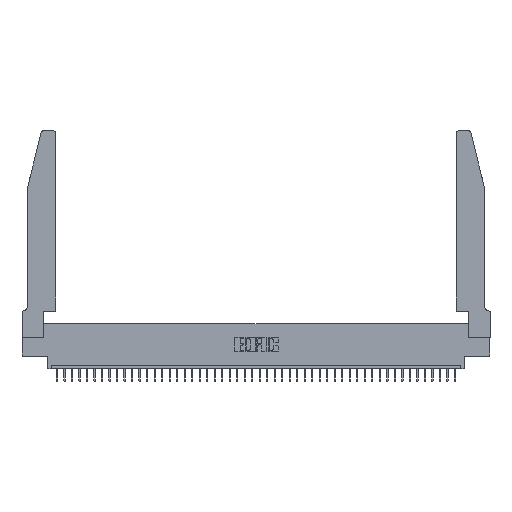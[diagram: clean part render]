
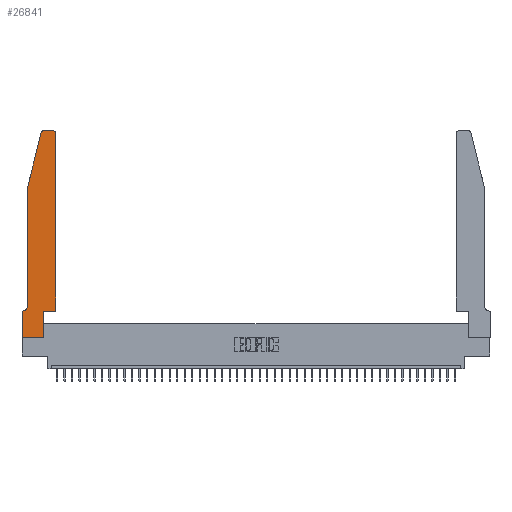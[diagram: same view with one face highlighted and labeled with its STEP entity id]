
A CAD part, top view. The second image highlights one B-rep face of the part: STEP entity #26841.
In plain terms, the highlighted planar face has unit normal (0, 0, 1).
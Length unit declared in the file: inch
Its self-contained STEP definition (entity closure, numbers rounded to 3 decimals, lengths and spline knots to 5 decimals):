
#531 = DIRECTION ( 'NONE',  ( 1., 0., 0. ) ) ;
#1023 = ORIENTED_EDGE ( 'NONE', *, *, #35085, .T. ) ;
#1380 = VERTEX_POINT ( 'NONE', #29385 ) ;
#1399 = VECTOR ( 'NONE', #27630, 39.37008 ) ;
#1460 = CARTESIAN_POINT ( 'NONE',  ( 0.0055, 0.42, 0.37 ) ) ;
#1509 = CARTESIAN_POINT ( 'NONE',  ( 0.284, 2.72, 0.37 ) ) ;
#1550 = CARTESIAN_POINT ( 'NONE',  ( 0.0755, 0.35, 0.37 ) ) ;
#1825 = VECTOR ( 'NONE', #17732, 39.37008 ) ;
#2286 = VERTEX_POINT ( 'NONE', #15661 ) ;
#3077 = CARTESIAN_POINT ( 'NONE',  ( 0.2865, 0.35, 0.37 ) ) ;
#3195 = ORIENTED_EDGE ( 'NONE', *, *, #18714, .T. ) ;
#3375 = ORIENTED_EDGE ( 'NONE', *, *, #33990, .T. ) ;
#3528 = PLANE ( 'NONE',  #32171 ) ;
#4137 = ORIENTED_EDGE ( 'NONE', *, *, #41520, .T. ) ;
#4184 = ORIENTED_EDGE ( 'NONE', *, *, #13365, .T. ) ;
#4264 = VERTEX_POINT ( 'NONE', #23359 ) ;
#4670 = CARTESIAN_POINT ( 'NONE',  ( 0.284, 2.75, 0.37 ) ) ;
#5471 = ORIENTED_EDGE ( 'NONE', *, *, #19715, .T. ) ;
#6332 = VECTOR ( 'NONE', #34596, 39.37008 ) ;
#7125 = EDGE_CURVE ( 'NONE', #2286, #23668, #32924, .T. ) ;
#8430 = DIRECTION ( 'NONE',  ( -1., 0., 0. ) ) ;
#8462 = DIRECTION ( 'NONE',  ( 1., 0., 0. ) ) ;
#10870 = VERTEX_POINT ( 'NONE', #19132 ) ;
#11763 = DIRECTION ( 'NONE',  ( 0., 0., 1. ) ) ;
#12128 = VECTOR ( 'NONE', #14571, 39.37008 ) ;
#12624 = VERTEX_POINT ( 'NONE', #4670 ) ;
#13365 = EDGE_CURVE ( 'NONE', #4264, #10870, #25734, .T. ) ;
#13976 = CARTESIAN_POINT ( 'NONE',  ( 0.2865, 0., 0.37 ) ) ;
#14091 = DIRECTION ( 'NONE',  ( 1., 0., 0. ) ) ;
#14571 = DIRECTION ( 'NONE',  ( 0., 1., 0. ) ) ;
#14810 = VERTEX_POINT ( 'NONE', #31232 ) ;
#14956 = VECTOR ( 'NONE', #15767, 39.37008 ) ;
#15661 = CARTESIAN_POINT ( 'NONE',  ( 0., 0.35, 0.37 ) ) ;
#15767 = DIRECTION ( 'NONE',  ( 0., -1., 0. ) ) ;
#16477 = EDGE_CURVE ( 'NONE', #14810, #12624, #29473, .T. ) ;
#16631 = FACE_OUTER_BOUND ( 'NONE', #20950, .T. ) ;
#17285 = VERTEX_POINT ( 'NONE', #38273 ) ;
#17711 = CARTESIAN_POINT ( 'NONE',  ( 0.4505, 0.35, 0.37 ) ) ;
#17732 = DIRECTION ( 'NONE',  ( -1., 0., 0. ) ) ;
#18138 = CARTESIAN_POINT ( 'NONE',  ( 0.0755, 2., 0.37 ) ) ;
#18714 = EDGE_CURVE ( 'NONE', #17285, #14810, #20323, .T. ) ;
#19132 = CARTESIAN_POINT ( 'NONE',  ( 0.0055, 0.35, 0.37 ) ) ;
#19475 = LINE ( 'NONE', #18138, #24700 ) ;
#19620 = EDGE_CURVE ( 'NONE', #10870, #2286, #42398, .T. ) ;
#19715 = EDGE_CURVE ( 'NONE', #24317, #27236, #36018, .T. ) ;
#20323 = CIRCLE ( 'NONE', #25554, 0.03 ) ;
#20950 = EDGE_LOOP ( 'NONE', ( #22391, #40862, #4137, #21047, #4184, #28801, #35682, #3375, #5471, #30517, #1023, #3195 ) ) ;
#21047 = ORIENTED_EDGE ( 'NONE', *, *, #34521, .T. ) ;
#21108 = CARTESIAN_POINT ( 'NONE',  ( 0.2605, 2.75, 0.37 ) ) ;
#22391 = ORIENTED_EDGE ( 'NONE', *, *, #16477, .T. ) ;
#23034 = CARTESIAN_POINT ( 'NONE',  ( 0.2865, 0.35, 0.37 ) ) ;
#23359 = CARTESIAN_POINT ( 'NONE',  ( 0.0755, 0.42, 0.37 ) ) ;
#23398 = VECTOR ( 'NONE', #14091, 39.37008 ) ;
#23668 = VERTEX_POINT ( 'NONE', #39765 ) ;
#23882 = VECTOR ( 'NONE', #8430, 39.37008 ) ;
#24177 = CARTESIAN_POINT ( 'NONE',  ( 0., 0.35, 0.37 ) ) ;
#24317 = VERTEX_POINT ( 'NONE', #13976 ) ;
#24516 = CARTESIAN_POINT ( 'NONE',  ( 0.4505, 0.35, 0.37 ) ) ;
#24700 = VECTOR ( 'NONE', #31941, 39.37008 ) ;
#25064 = DIRECTION ( 'NONE',  ( -1., 0., 0. ) ) ;
#25554 = AXIS2_PLACEMENT_3D ( 'NONE', #38648, #11763, #8462 ) ;
#25734 = CIRCLE ( 'NONE', #28755, 0.07 ) ;
#25797 = EDGE_CURVE ( 'NONE', #12624, #27061, #40508, .T. ) ;
#26274 = CARTESIAN_POINT ( 'NONE',  ( 0., 0., 0.37 ) ) ;
#26586 = LINE ( 'NONE', #30768, #23398 ) ;
#26841 = ADVANCED_FACE ( 'NONE', ( #16631 ), #3528, .T. ) ;
#27061 = VERTEX_POINT ( 'NONE', #39706 ) ;
#27140 = AXIS2_PLACEMENT_3D ( 'NONE', #1509, #38876, #28854 ) ;
#27236 = VERTEX_POINT ( 'NONE', #3077 ) ;
#27322 = DIRECTION ( 'NONE',  ( 0., 0., 1. ) ) ;
#27356 = CARTESIAN_POINT ( 'NONE',  ( 0.4505, 0.35, 0.37 ) ) ;
#27630 = DIRECTION ( 'NONE',  ( 1., 0., 0. ) ) ;
#28755 = AXIS2_PLACEMENT_3D ( 'NONE', #1460, #37054, #25064 ) ;
#28801 = ORIENTED_EDGE ( 'NONE', *, *, #19620, .T. ) ;
#28854 = DIRECTION ( 'NONE',  ( 1., 0., 0. ) ) ;
#29385 = CARTESIAN_POINT ( 'NONE',  ( 0.0755, 2., 0.37 ) ) ;
#29473 = LINE ( 'NONE', #21108, #1825 ) ;
#30517 = ORIENTED_EDGE ( 'NONE', *, *, #40677, .T. ) ;
#30691 = VECTOR ( 'NONE', #36013, 39.37008 ) ;
#30768 = CARTESIAN_POINT ( 'NONE',  ( 0., 0., 0.37 ) ) ;
#31232 = CARTESIAN_POINT ( 'NONE',  ( 0.4205, 2.75, 0.37 ) ) ;
#31941 = DIRECTION ( 'NONE',  ( -0.239, -0.971, 0. ) ) ;
#32171 = AXIS2_PLACEMENT_3D ( 'NONE', #24177, #27322, #531 ) ;
#32924 = LINE ( 'NONE', #26274, #14956 ) ;
#33990 = EDGE_CURVE ( 'NONE', #23668, #24317, #26586, .T. ) ;
#34521 = EDGE_CURVE ( 'NONE', #1380, #4264, #38099, .T. ) ;
#34596 = DIRECTION ( 'NONE',  ( 0., 1., 0. ) ) ;
#35085 = EDGE_CURVE ( 'NONE', #36410, #17285, #41211, .T. ) ;
#35682 = ORIENTED_EDGE ( 'NONE', *, *, #7125, .T. ) ;
#36013 = DIRECTION ( 'NONE',  ( 0., -1., 0. ) ) ;
#36018 = LINE ( 'NONE', #23034, #6332 ) ;
#36410 = VERTEX_POINT ( 'NONE', #24516 ) ;
#37054 = DIRECTION ( 'NONE',  ( 0., 0., -1. ) ) ;
#37502 = LINE ( 'NONE', #27356, #1399 ) ;
#38099 = LINE ( 'NONE', #39454, #30691 ) ;
#38273 = CARTESIAN_POINT ( 'NONE',  ( 0.4505, 2.72, 0.37 ) ) ;
#38648 = CARTESIAN_POINT ( 'NONE',  ( 0.4205, 2.72, 0.37 ) ) ;
#38876 = DIRECTION ( 'NONE',  ( 0., 0., 1. ) ) ;
#39454 = CARTESIAN_POINT ( 'NONE',  ( 0.0755, 2., 0.37 ) ) ;
#39706 = CARTESIAN_POINT ( 'NONE',  ( 0.25487, 2.72718, 0.37 ) ) ;
#39765 = CARTESIAN_POINT ( 'NONE',  ( 0., 0., 0.37 ) ) ;
#40508 = CIRCLE ( 'NONE', #27140, 0.03 ) ;
#40677 = EDGE_CURVE ( 'NONE', #27236, #36410, #37502, .T. ) ;
#40862 = ORIENTED_EDGE ( 'NONE', *, *, #25797, .T. ) ;
#41211 = LINE ( 'NONE', #17711, #12128 ) ;
#41520 = EDGE_CURVE ( 'NONE', #27061, #1380, #19475, .T. ) ;
#42398 = LINE ( 'NONE', #1550, #23882 ) ;
